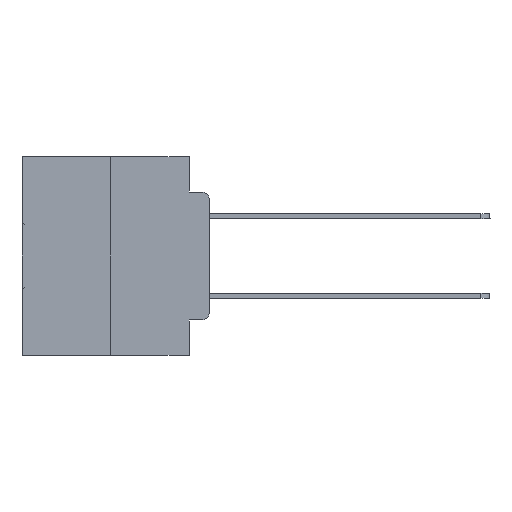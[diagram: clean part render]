
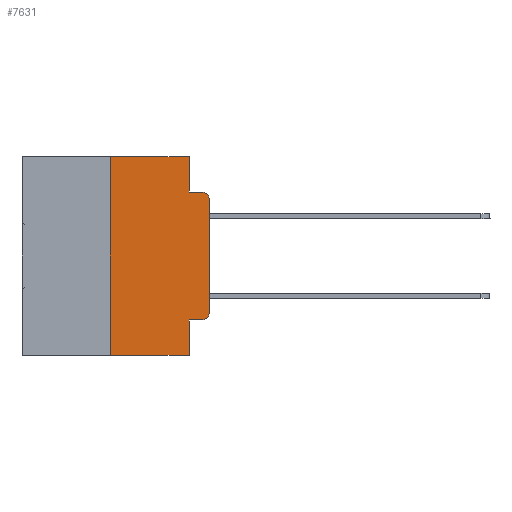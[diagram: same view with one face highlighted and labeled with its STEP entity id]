
A CAD part, left-side view. The second image highlights one B-rep face of the part: STEP entity #7631.
In plain terms, the highlighted planar face has unit normal (-1, 0, 0).
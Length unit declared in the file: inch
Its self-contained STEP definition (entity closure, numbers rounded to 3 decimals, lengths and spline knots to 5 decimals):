
#257 = DIRECTION ( 'NONE',  ( 0., 0., -1. ) ) ;
#282 = CARTESIAN_POINT ( 'NONE',  ( 0., 0.02, -0.4115 ) ) ;
#1365 = DIRECTION ( 'NONE',  ( 0., 0., -1. ) ) ;
#2848 = VERTEX_POINT ( 'NONE', #20863 ) ;
#2901 = CARTESIAN_POINT ( 'NONE',  ( 0., 0.02, -0.1085 ) ) ;
#2917 = FACE_OUTER_BOUND ( 'NONE', #4560, .T. ) ;
#3423 = ORIENTED_EDGE ( 'NONE', *, *, #8476, .F. ) ;
#3999 = VERTEX_POINT ( 'NONE', #282 ) ;
#4279 = ORIENTED_EDGE ( 'NONE', *, *, #28513, .F. ) ;
#4560 = EDGE_LOOP ( 'NONE', ( #5490, #30422, #4279, #11117, #27258, #3423, #6345, #14608, #20000, #29436 ) ) ;
#4646 = VERTEX_POINT ( 'NONE', #6894 ) ;
#5210 = DIRECTION ( 'NONE',  ( 0., -1., 0. ) ) ;
#5263 = EDGE_CURVE ( 'NONE', #28691, #26723, #29977, .T. ) ;
#5409 = VERTEX_POINT ( 'NONE', #9761 ) ;
#5459 = DIRECTION ( 'NONE',  ( -1., 0., 0. ) ) ;
#5490 = ORIENTED_EDGE ( 'NONE', *, *, #25995, .T. ) ;
#5923 = CIRCLE ( 'NONE', #16965, 0.02 ) ;
#5991 = VECTOR ( 'NONE', #14098, 39.37008 ) ;
#6344 = VECTOR ( 'NONE', #17194, 39.37008 ) ;
#6345 = ORIENTED_EDGE ( 'NONE', *, *, #5263, .T. ) ;
#6894 = CARTESIAN_POINT ( 'NONE',  ( 0., 0.051, -0.0885 ) ) ;
#6990 = LINE ( 'NONE', #15929, #23552 ) ;
#7017 = LINE ( 'NONE', #18975, #26907 ) ;
#7176 = CARTESIAN_POINT ( 'NONE',  ( 0., 0.051, 0. ) ) ;
#7462 = LINE ( 'NONE', #18660, #33955 ) ;
#7631 = ADVANCED_FACE ( 'NONE', ( #2917 ), #25802, .F. ) ;
#8000 = EDGE_CURVE ( 'NONE', #17088, #24436, #7462, .T. ) ;
#8432 = CARTESIAN_POINT ( 'NONE',  ( 0., 0.051, -0.5 ) ) ;
#8476 = EDGE_CURVE ( 'NONE', #28691, #17088, #6990, .T. ) ;
#9761 = CARTESIAN_POINT ( 'NONE',  ( 0., 0.051, -0.4115 ) ) ;
#9937 = DIRECTION ( 'NONE',  ( 1., 0., 0. ) ) ;
#10201 = DIRECTION ( 'NONE',  ( 0., 0., -1. ) ) ;
#10279 = VECTOR ( 'NONE', #21408, 39.37008 ) ;
#10449 = VECTOR ( 'NONE', #15410, 39.37008 ) ;
#11117 = ORIENTED_EDGE ( 'NONE', *, *, #31953, .F. ) ;
#12171 = CARTESIAN_POINT ( 'NONE',  ( 0., 0.02, -0.3915 ) ) ;
#13606 = LINE ( 'NONE', #16099, #10279 ) ;
#13614 = AXIS2_PLACEMENT_3D ( 'NONE', #28556, #9937, #33753 ) ;
#13776 = CARTESIAN_POINT ( 'NONE',  ( 0., 0., -0.3915 ) ) ;
#13863 = VECTOR ( 'NONE', #27823, 39.37008 ) ;
#14092 = CARTESIAN_POINT ( 'NONE',  ( 0., 0.25, -0.5 ) ) ;
#14098 = DIRECTION ( 'NONE',  ( 0., -1., 0. ) ) ;
#14284 = CARTESIAN_POINT ( 'NONE',  ( 0., 0., -0.1085 ) ) ;
#14508 = CARTESIAN_POINT ( 'NONE',  ( 0., 0.473, -0.5 ) ) ;
#14523 = AXIS2_PLACEMENT_3D ( 'NONE', #2901, #5459, #257 ) ;
#14608 = ORIENTED_EDGE ( 'NONE', *, *, #23425, .F. ) ;
#15410 = DIRECTION ( 'NONE',  ( 0., 0., 1. ) ) ;
#15929 = CARTESIAN_POINT ( 'NONE',  ( 0., 0.25, 0. ) ) ;
#16099 = CARTESIAN_POINT ( 'NONE',  ( 0., 0.051, -0.0885 ) ) ;
#16413 = CIRCLE ( 'NONE', #14523, 0.02 ) ;
#16965 = AXIS2_PLACEMENT_3D ( 'NONE', #12171, #30647, #1365 ) ;
#17088 = VERTEX_POINT ( 'NONE', #20820 ) ;
#17194 = DIRECTION ( 'NONE',  ( 0., 0., -1. ) ) ;
#18660 = CARTESIAN_POINT ( 'NONE',  ( 0., 0.473, 0. ) ) ;
#18975 = CARTESIAN_POINT ( 'NONE',  ( 0., 0.051, 0. ) ) ;
#19159 = LINE ( 'NONE', #20835, #10449 ) ;
#20000 = ORIENTED_EDGE ( 'NONE', *, *, #20483, .T. ) ;
#20333 = EDGE_CURVE ( 'NONE', #31961, #2848, #16413, .T. ) ;
#20483 = EDGE_CURVE ( 'NONE', #5409, #3999, #24218, .T. ) ;
#20820 = CARTESIAN_POINT ( 'NONE',  ( 0., 0.25, 0. ) ) ;
#20835 = CARTESIAN_POINT ( 'NONE',  ( 0., 0., 0. ) ) ;
#20863 = CARTESIAN_POINT ( 'NONE',  ( 0., 0.02, -0.0885 ) ) ;
#21408 = DIRECTION ( 'NONE',  ( 0., -1., 0. ) ) ;
#22367 = CARTESIAN_POINT ( 'NONE',  ( 0., 0.051, 0. ) ) ;
#23425 = EDGE_CURVE ( 'NONE', #5409, #26723, #7017, .T. ) ;
#23552 = VECTOR ( 'NONE', #29535, 39.37008 ) ;
#24218 = LINE ( 'NONE', #32162, #5991 ) ;
#24436 = VERTEX_POINT ( 'NONE', #7176 ) ;
#25802 = PLANE ( 'NONE',  #13614 ) ;
#25850 = EDGE_CURVE ( 'NONE', #3999, #29374, #5923, .T. ) ;
#25995 = EDGE_CURVE ( 'NONE', #29374, #31961, #19159, .T. ) ;
#26723 = VERTEX_POINT ( 'NONE', #8432 ) ;
#26907 = VECTOR ( 'NONE', #10201, 39.37008 ) ;
#27258 = ORIENTED_EDGE ( 'NONE', *, *, #8000, .F. ) ;
#27823 = DIRECTION ( 'NONE',  ( 0., -1., 0. ) ) ;
#28513 = EDGE_CURVE ( 'NONE', #4646, #2848, #13606, .T. ) ;
#28556 = CARTESIAN_POINT ( 'NONE',  ( 0., 0.473, 0. ) ) ;
#28691 = VERTEX_POINT ( 'NONE', #14092 ) ;
#29374 = VERTEX_POINT ( 'NONE', #13776 ) ;
#29436 = ORIENTED_EDGE ( 'NONE', *, *, #25850, .T. ) ;
#29535 = DIRECTION ( 'NONE',  ( 0., 0., 1. ) ) ;
#29936 = LINE ( 'NONE', #22367, #6344 ) ;
#29977 = LINE ( 'NONE', #14508, #13863 ) ;
#30422 = ORIENTED_EDGE ( 'NONE', *, *, #20333, .T. ) ;
#30647 = DIRECTION ( 'NONE',  ( -1., 0., 0. ) ) ;
#31953 = EDGE_CURVE ( 'NONE', #24436, #4646, #29936, .T. ) ;
#31961 = VERTEX_POINT ( 'NONE', #14284 ) ;
#32162 = CARTESIAN_POINT ( 'NONE',  ( 0., 0.051, -0.4115 ) ) ;
#33753 = DIRECTION ( 'NONE',  ( 0., 0., -1. ) ) ;
#33955 = VECTOR ( 'NONE', #5210, 39.37008 ) ;
